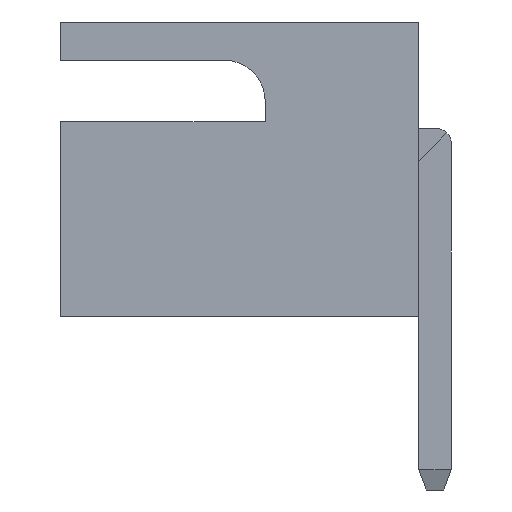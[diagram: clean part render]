
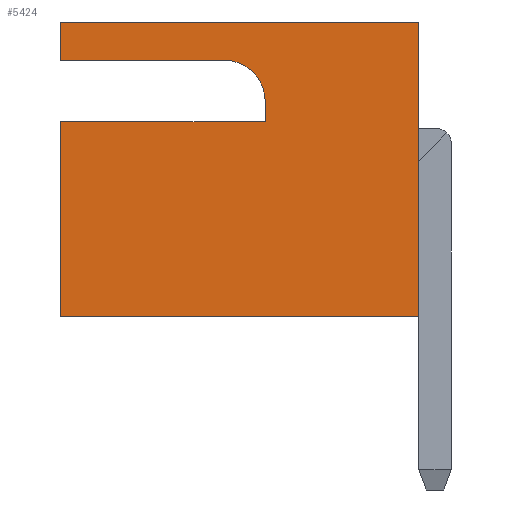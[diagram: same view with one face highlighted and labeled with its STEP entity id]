
A CAD part, left-side view. The second image highlights one B-rep face of the part: STEP entity #5424.
In plain terms, the highlighted planar face has unit normal (-1, 0, 0).
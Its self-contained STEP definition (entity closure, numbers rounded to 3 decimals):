
#60 = CARTESIAN_POINT ( 'NONE',  ( -12.5, 3.8, 1.325 ) ) ;
#62 = ORIENTED_EDGE ( 'NONE', *, *, #5055, .F. ) ;
#133 = CARTESIAN_POINT ( 'NONE',  ( -12.5, 7., -2.875 ) ) ;
#144 = DIRECTION ( 'NONE',  ( 0., 0., -1. ) ) ;
#224 = VERTEX_POINT ( 'NONE', #4008 ) ;
#283 = VECTOR ( 'NONE', #3290, 1000. ) ;
#326 = LINE ( 'NONE', #1569, #3599 ) ;
#402 = ORIENTED_EDGE ( 'NONE', *, *, #2737, .F. ) ;
#560 = VERTEX_POINT ( 'NONE', #2084 ) ;
#637 = CARTESIAN_POINT ( 'NONE',  ( -12.5, 7., 0.925 ) ) ;
#684 = EDGE_CURVE ( 'NONE', #224, #2835, #4335, .T. ) ;
#764 = ORIENTED_EDGE ( 'NONE', *, *, #1930, .T. ) ;
#915 = DIRECTION ( 'NONE',  ( 0., 0., 1. ) ) ;
#937 = EDGE_LOOP ( 'NONE', ( #2514, #1624, #1272, #3229, #764, #402, #2189, #1062, #62 ) ) ;
#982 = EDGE_CURVE ( 'NONE', #2835, #3357, #326, .T. ) ;
#1002 = VERTEX_POINT ( 'NONE', #1129 ) ;
#1062 = ORIENTED_EDGE ( 'NONE', *, *, #982, .T. ) ;
#1129 = CARTESIAN_POINT ( 'NONE',  ( -12.5, 7., 2.125 ) ) ;
#1272 = ORIENTED_EDGE ( 'NONE', *, *, #2362, .T. ) ;
#1479 = AXIS2_PLACEMENT_3D ( 'NONE', #60, #1724, #144 ) ;
#1501 = VERTEX_POINT ( 'NONE', #1903 ) ;
#1569 = CARTESIAN_POINT ( 'NONE',  ( -12.5, 0., -2.875 ) ) ;
#1580 = VECTOR ( 'NONE', #915, 1000. ) ;
#1624 = ORIENTED_EDGE ( 'NONE', *, *, #4067, .T. ) ;
#1724 = DIRECTION ( 'NONE',  ( 1., 0., 0. ) ) ;
#1849 = LINE ( 'NONE', #637, #5395 ) ;
#1892 = VECTOR ( 'NONE', #2573, 1000. ) ;
#1903 = CARTESIAN_POINT ( 'NONE',  ( -12.5, 3.8, 2.125 ) ) ;
#1930 = EDGE_CURVE ( 'NONE', #3244, #3130, #1849, .T. ) ;
#1944 = LINE ( 'NONE', #3632, #1892 ) ;
#2017 = VECTOR ( 'NONE', #5433, 1000. ) ;
#2023 = CARTESIAN_POINT ( 'NONE',  ( -12.5, 7., 2.875 ) ) ;
#2084 = CARTESIAN_POINT ( 'NONE',  ( -12.5, 3., 1.325 ) ) ;
#2189 = ORIENTED_EDGE ( 'NONE', *, *, #684, .T. ) ;
#2252 = FACE_OUTER_BOUND ( 'NONE', #937, .T. ) ;
#2362 = EDGE_CURVE ( 'NONE', #1501, #560, #4132, .T. ) ;
#2390 = CARTESIAN_POINT ( 'NONE',  ( -12.5, 0., 2.875 ) ) ;
#2398 = AXIS2_PLACEMENT_3D ( 'NONE', #3569, #2805, #3144 ) ;
#2479 = CARTESIAN_POINT ( 'NONE',  ( -12.5, 7., 0.925 ) ) ;
#2514 = ORIENTED_EDGE ( 'NONE', *, *, #4607, .F. ) ;
#2573 = DIRECTION ( 'NONE',  ( 0., -1., 0. ) ) ;
#2597 = LINE ( 'NONE', #4664, #3870 ) ;
#2611 = DIRECTION ( 'NONE',  ( 0., -1., 0. ) ) ;
#2688 = CARTESIAN_POINT ( 'NONE',  ( -12.5, 7., -2.875 ) ) ;
#2737 = EDGE_CURVE ( 'NONE', #224, #3130, #2597, .T. ) ;
#2805 = DIRECTION ( 'NONE',  ( 1., 0., 0. ) ) ;
#2835 = VERTEX_POINT ( 'NONE', #4958 ) ;
#2895 = DIRECTION ( 'NONE',  ( 0., 0., 1. ) ) ;
#2899 = LINE ( 'NONE', #2023, #283 ) ;
#3044 = DIRECTION ( 'NONE',  ( 0., 0., 1. ) ) ;
#3130 = VERTEX_POINT ( 'NONE', #2479 ) ;
#3144 = DIRECTION ( 'NONE',  ( 0., 0., -1. ) ) ;
#3229 = ORIENTED_EDGE ( 'NONE', *, *, #5149, .T. ) ;
#3244 = VERTEX_POINT ( 'NONE', #3964 ) ;
#3290 = DIRECTION ( 'NONE',  ( 0., -1., 0. ) ) ;
#3325 = VECTOR ( 'NONE', #2611, 1000. ) ;
#3357 = VERTEX_POINT ( 'NONE', #2390 ) ;
#3535 = DIRECTION ( 'NONE',  ( 0., 1., 0. ) ) ;
#3569 = CARTESIAN_POINT ( 'NONE',  ( -12.5, 7., -2.875 ) ) ;
#3599 = VECTOR ( 'NONE', #2895, 1000. ) ;
#3632 = CARTESIAN_POINT ( 'NONE',  ( -12.5, 7., 2.125 ) ) ;
#3661 = CARTESIAN_POINT ( 'NONE',  ( -12.5, 7., 2.875 ) ) ;
#3870 = VECTOR ( 'NONE', #3044, 1000. ) ;
#3964 = CARTESIAN_POINT ( 'NONE',  ( -12.5, 3., 0.925 ) ) ;
#3974 = VERTEX_POINT ( 'NONE', #3661 ) ;
#4008 = CARTESIAN_POINT ( 'NONE',  ( -12.5, 7., -2.875 ) ) ;
#4029 = PLANE ( 'NONE',  #2398 ) ;
#4067 = EDGE_CURVE ( 'NONE', #1002, #1501, #1944, .T. ) ;
#4132 = CIRCLE ( 'NONE', #1479, 0.8 ) ;
#4335 = LINE ( 'NONE', #2688, #3325 ) ;
#4607 = EDGE_CURVE ( 'NONE', #1002, #3974, #4720, .T. ) ;
#4659 = CARTESIAN_POINT ( 'NONE',  ( -12.5, 3., 1.325 ) ) ;
#4664 = CARTESIAN_POINT ( 'NONE',  ( -12.5, 7., -2.875 ) ) ;
#4720 = LINE ( 'NONE', #133, #1580 ) ;
#4958 = CARTESIAN_POINT ( 'NONE',  ( -12.5, 0., -2.875 ) ) ;
#5055 = EDGE_CURVE ( 'NONE', #3974, #3357, #2899, .T. ) ;
#5062 = LINE ( 'NONE', #4659, #2017 ) ;
#5149 = EDGE_CURVE ( 'NONE', #560, #3244, #5062, .T. ) ;
#5395 = VECTOR ( 'NONE', #3535, 1000. ) ;
#5424 = ADVANCED_FACE ( 'NONE', ( #2252 ), #4029, .F. ) ;
#5433 = DIRECTION ( 'NONE',  ( 0., 0., -1. ) ) ;
